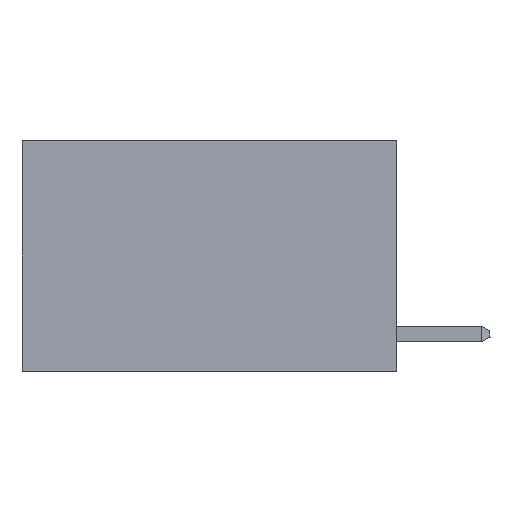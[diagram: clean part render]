
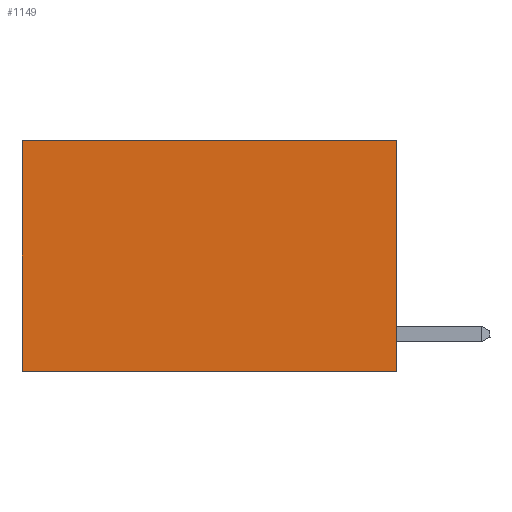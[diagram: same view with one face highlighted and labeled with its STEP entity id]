
A CAD part, left-side view. The second image highlights one B-rep face of the part: STEP entity #1149.
In plain terms, the highlighted planar face has unit normal (-1, 0, 0).
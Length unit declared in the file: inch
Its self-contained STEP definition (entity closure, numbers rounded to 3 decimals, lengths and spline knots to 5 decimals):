
#1149 = ADVANCED_FACE ( 'NONE', ( #6755 ), #24699, .F. ) ;
#1223 = EDGE_LOOP ( 'NONE', ( #25219, #7079, #16848, #10059 ) ) ;
#1768 = VERTEX_POINT ( 'NONE', #12401 ) ;
#1921 = LINE ( 'NONE', #19062, #12133 ) ;
#2425 = DIRECTION ( 'NONE',  ( 0., 0., -1. ) ) ;
#3141 = VERTEX_POINT ( 'NONE', #4377 ) ;
#4035 = VECTOR ( 'NONE', #11104, 39.37008 ) ;
#4052 = AXIS2_PLACEMENT_3D ( 'NONE', #12608, #14634, #2425 ) ;
#4377 = CARTESIAN_POINT ( 'NONE',  ( 0.2625, 0., 0. ) ) ;
#4549 = CARTESIAN_POINT ( 'NONE',  ( 0.2625, 0., -0.37 ) ) ;
#5807 = VERTEX_POINT ( 'NONE', #13189 ) ;
#6566 = CARTESIAN_POINT ( 'NONE',  ( 0.2625, 0.6, 0. ) ) ;
#6755 = FACE_OUTER_BOUND ( 'NONE', #1223, .T. ) ;
#7079 = ORIENTED_EDGE ( 'NONE', *, *, #17679, .F. ) ;
#10059 = ORIENTED_EDGE ( 'NONE', *, *, #25872, .T. ) ;
#11104 = DIRECTION ( 'NONE',  ( 0., 1., 0. ) ) ;
#12133 = VECTOR ( 'NONE', #23090, 39.37008 ) ;
#12401 = CARTESIAN_POINT ( 'NONE',  ( 0.2625, 0.6, 0. ) ) ;
#12608 = CARTESIAN_POINT ( 'NONE',  ( 0.2625, 0., 0. ) ) ;
#13156 = CARTESIAN_POINT ( 'NONE',  ( 0.2625, 0., 0. ) ) ;
#13189 = CARTESIAN_POINT ( 'NONE',  ( 0.2625, 0.6, -0.37 ) ) ;
#13671 = LINE ( 'NONE', #6566, #19118 ) ;
#14634 = DIRECTION ( 'NONE',  ( 1., 0., 0. ) ) ;
#15524 = LINE ( 'NONE', #13156, #4035 ) ;
#16199 = VERTEX_POINT ( 'NONE', #26013 ) ;
#16848 = ORIENTED_EDGE ( 'NONE', *, *, #24037, .F. ) ;
#17059 = DIRECTION ( 'NONE',  ( 0., 0., -1. ) ) ;
#17679 = EDGE_CURVE ( 'NONE', #16199, #5807, #22161, .T. ) ;
#18093 = VECTOR ( 'NONE', #18835, 39.37008 ) ;
#18835 = DIRECTION ( 'NONE',  ( 0., 1., 0. ) ) ;
#19062 = CARTESIAN_POINT ( 'NONE',  ( 0.2625, 0., 0. ) ) ;
#19118 = VECTOR ( 'NONE', #17059, 39.37008 ) ;
#22161 = LINE ( 'NONE', #4549, #18093 ) ;
#23090 = DIRECTION ( 'NONE',  ( 0., 0., -1. ) ) ;
#24037 = EDGE_CURVE ( 'NONE', #3141, #16199, #1921, .T. ) ;
#24622 = EDGE_CURVE ( 'NONE', #1768, #5807, #13671, .T. ) ;
#24699 = PLANE ( 'NONE',  #4052 ) ;
#25219 = ORIENTED_EDGE ( 'NONE', *, *, #24622, .T. ) ;
#25872 = EDGE_CURVE ( 'NONE', #3141, #1768, #15524, .T. ) ;
#26013 = CARTESIAN_POINT ( 'NONE',  ( 0.2625, 0., -0.37 ) ) ;
